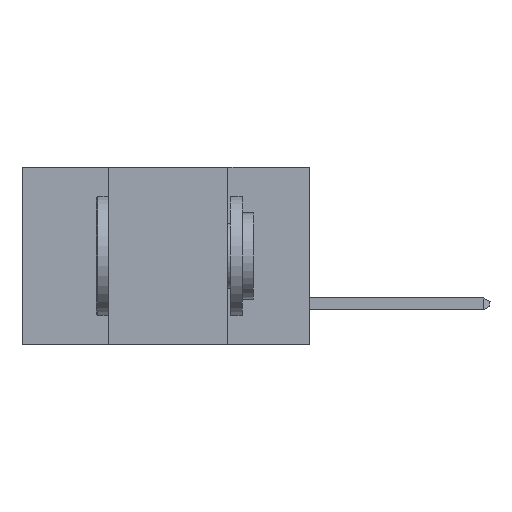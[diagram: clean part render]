
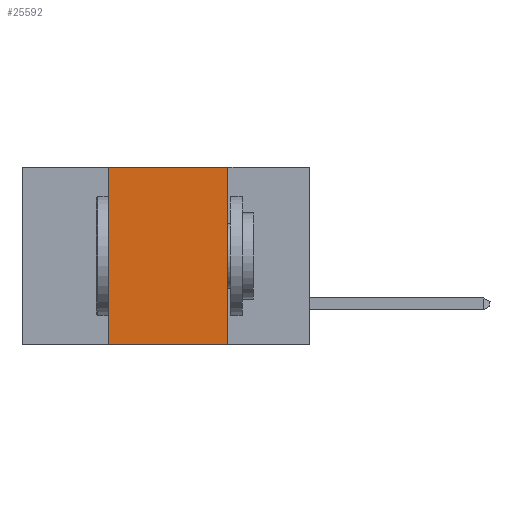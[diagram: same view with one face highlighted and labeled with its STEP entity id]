
A CAD part, left-side view. The second image highlights one B-rep face of the part: STEP entity #25592.
In plain terms, the highlighted planar face has unit normal (-1, 0, 0).
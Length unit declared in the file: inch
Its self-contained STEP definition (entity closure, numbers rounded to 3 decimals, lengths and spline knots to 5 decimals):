
#101 = DIRECTION ( 'NONE',  ( 0., 0., 1. ) ) ;
#1375 = AXIS2_PLACEMENT_3D ( 'NONE', #19916, #3404, #17478 ) ;
#1882 = FACE_OUTER_BOUND ( 'NONE', #21768, .T. ) ;
#2168 = ORIENTED_EDGE ( 'NONE', *, *, #28038, .F. ) ;
#2193 = CARTESIAN_POINT ( 'NONE',  ( 0., 0.42, -0.37 ) ) ;
#2788 = ORIENTED_EDGE ( 'NONE', *, *, #8114, .F. ) ;
#3404 = DIRECTION ( 'NONE',  ( 1., 0., 0. ) ) ;
#3482 = VECTOR ( 'NONE', #15693, 39.37008 ) ;
#4082 = CARTESIAN_POINT ( 'NONE',  ( 0., 0.17, 0. ) ) ;
#4953 = LINE ( 'NONE', #8994, #3482 ) ;
#6133 = CARTESIAN_POINT ( 'NONE',  ( 0., 0.6, 0. ) ) ;
#8114 = EDGE_CURVE ( 'NONE', #28191, #14556, #8760, .T. ) ;
#8760 = LINE ( 'NONE', #23724, #20560 ) ;
#8994 = CARTESIAN_POINT ( 'NONE',  ( 0., 0.6, -0.37 ) ) ;
#10008 = ORIENTED_EDGE ( 'NONE', *, *, #11520, .T. ) ;
#10654 = LINE ( 'NONE', #4082, #28628 ) ;
#11520 = EDGE_CURVE ( 'NONE', #28191, #19111, #4953, .T. ) ;
#11894 = LINE ( 'NONE', #6133, #29181 ) ;
#12667 = EDGE_CURVE ( 'NONE', #14556, #21937, #11894, .T. ) ;
#14556 = VERTEX_POINT ( 'NONE', #14879 ) ;
#14879 = CARTESIAN_POINT ( 'NONE',  ( 0., 0.42, 0. ) ) ;
#15693 = DIRECTION ( 'NONE',  ( 0., -1., 0. ) ) ;
#16946 = CARTESIAN_POINT ( 'NONE',  ( 0., 0.17, 0. ) ) ;
#17073 = ORIENTED_EDGE ( 'NONE', *, *, #12667, .F. ) ;
#17478 = DIRECTION ( 'NONE',  ( 0., 0., -1. ) ) ;
#19111 = VERTEX_POINT ( 'NONE', #19661 ) ;
#19513 = PLANE ( 'NONE',  #1375 ) ;
#19661 = CARTESIAN_POINT ( 'NONE',  ( 0., 0.17, -0.37 ) ) ;
#19916 = CARTESIAN_POINT ( 'NONE',  ( 0., 0.6, 0. ) ) ;
#20560 = VECTOR ( 'NONE', #101, 39.37008 ) ;
#20598 = DIRECTION ( 'NONE',  ( 0., 0., -1. ) ) ;
#21768 = EDGE_LOOP ( 'NONE', ( #2168, #17073, #2788, #10008 ) ) ;
#21937 = VERTEX_POINT ( 'NONE', #16946 ) ;
#23724 = CARTESIAN_POINT ( 'NONE',  ( 0., 0.42, 0. ) ) ;
#25115 = DIRECTION ( 'NONE',  ( 0., -1., 0. ) ) ;
#25592 = ADVANCED_FACE ( 'NONE', ( #1882 ), #19513, .F. ) ;
#28038 = EDGE_CURVE ( 'NONE', #21937, #19111, #10654, .T. ) ;
#28191 = VERTEX_POINT ( 'NONE', #2193 ) ;
#28628 = VECTOR ( 'NONE', #20598, 39.37008 ) ;
#29181 = VECTOR ( 'NONE', #25115, 39.37008 ) ;
